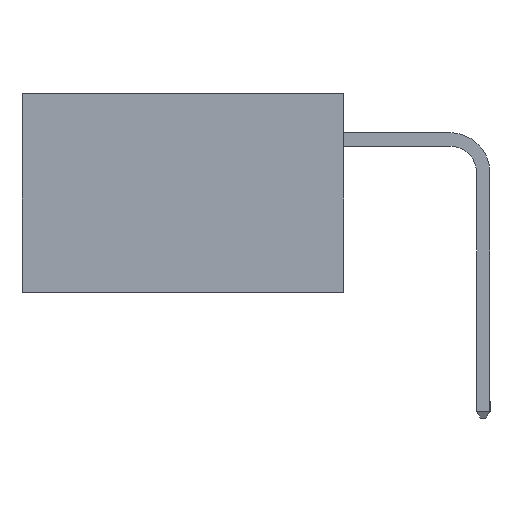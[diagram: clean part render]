
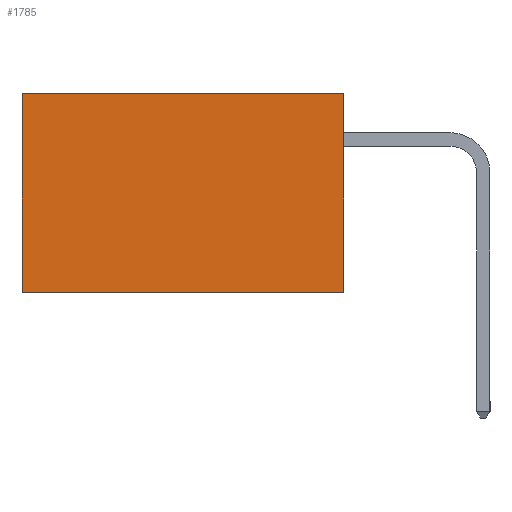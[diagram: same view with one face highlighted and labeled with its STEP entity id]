
A CAD part, left-side view. The second image highlights one B-rep face of the part: STEP entity #1785.
In plain terms, the highlighted planar face has unit normal (-1, 0, 0).
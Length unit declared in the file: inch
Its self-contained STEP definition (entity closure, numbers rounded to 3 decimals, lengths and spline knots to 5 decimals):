
#286 = DIRECTION ( 'NONE',  ( 0., 1., 0. ) ) ;
#989 = VERTEX_POINT ( 'NONE', #8114 ) ;
#1757 = CARTESIAN_POINT ( 'NONE',  ( 0.2615, 0.6, -0.37 ) ) ;
#1785 = ADVANCED_FACE ( 'NONE', ( #11135 ), #8877, .F. ) ;
#1934 = VECTOR ( 'NONE', #286, 39.37008 ) ;
#2001 = VECTOR ( 'NONE', #7732, 39.37008 ) ;
#2047 = DIRECTION ( 'NONE',  ( 0., 0., -1. ) ) ;
#2160 = VERTEX_POINT ( 'NONE', #7964 ) ;
#2435 = LINE ( 'NONE', #8833, #1934 ) ;
#2458 = CARTESIAN_POINT ( 'NONE',  ( 0.2615, 0., -0.37 ) ) ;
#2721 = EDGE_CURVE ( 'NONE', #989, #2786, #4682, .T. ) ;
#2765 = DIRECTION ( 'NONE',  ( 0., 0., -1. ) ) ;
#2786 = VERTEX_POINT ( 'NONE', #11411 ) ;
#3553 = EDGE_CURVE ( 'NONE', #2786, #12561, #4162, .T. ) ;
#3579 = CARTESIAN_POINT ( 'NONE',  ( 0.2615, 0., -0.37 ) ) ;
#3641 = VECTOR ( 'NONE', #4314, 39.37008 ) ;
#4162 = LINE ( 'NONE', #12885, #3641 ) ;
#4314 = DIRECTION ( 'NONE',  ( 0., 1., 0. ) ) ;
#4682 = LINE ( 'NONE', #3579, #2001 ) ;
#4749 = VECTOR ( 'NONE', #2047, 39.37008 ) ;
#5102 = ORIENTED_EDGE ( 'NONE', *, *, #3553, .F. ) ;
#5578 = EDGE_LOOP ( 'NONE', ( #13319, #5102, #6627, #9633 ) ) ;
#6627 = ORIENTED_EDGE ( 'NONE', *, *, #2721, .F. ) ;
#6792 = AXIS2_PLACEMENT_3D ( 'NONE', #2458, #9061, #2765 ) ;
#7732 = DIRECTION ( 'NONE',  ( 0., 0., -1. ) ) ;
#7964 = CARTESIAN_POINT ( 'NONE',  ( 0.2615, 0.6, 0. ) ) ;
#8114 = CARTESIAN_POINT ( 'NONE',  ( 0.2615, 0., 0. ) ) ;
#8833 = CARTESIAN_POINT ( 'NONE',  ( 0.2615, 0., 0. ) ) ;
#8877 = PLANE ( 'NONE',  #6792 ) ;
#9061 = DIRECTION ( 'NONE',  ( 1., 0., 0. ) ) ;
#9598 = CARTESIAN_POINT ( 'NONE',  ( 0.2615, 0.6, -0.37 ) ) ;
#9633 = ORIENTED_EDGE ( 'NONE', *, *, #10068, .T. ) ;
#10068 = EDGE_CURVE ( 'NONE', #989, #2160, #2435, .T. ) ;
#10555 = EDGE_CURVE ( 'NONE', #2160, #12561, #13852, .T. ) ;
#11135 = FACE_OUTER_BOUND ( 'NONE', #5578, .T. ) ;
#11411 = CARTESIAN_POINT ( 'NONE',  ( 0.2615, 0., -0.37 ) ) ;
#12561 = VERTEX_POINT ( 'NONE', #1757 ) ;
#12885 = CARTESIAN_POINT ( 'NONE',  ( 0.2615, 0., -0.37 ) ) ;
#13319 = ORIENTED_EDGE ( 'NONE', *, *, #10555, .T. ) ;
#13852 = LINE ( 'NONE', #9598, #4749 ) ;
